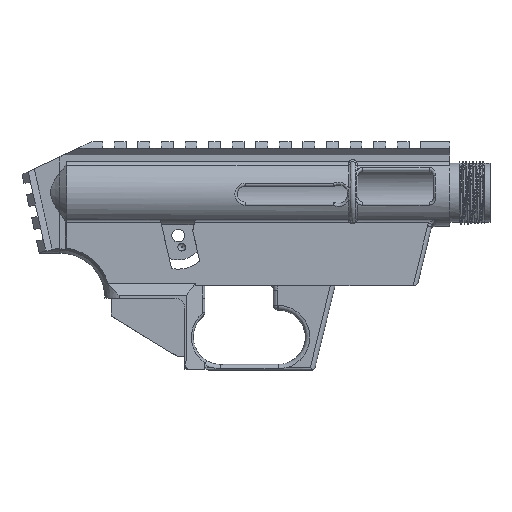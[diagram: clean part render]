
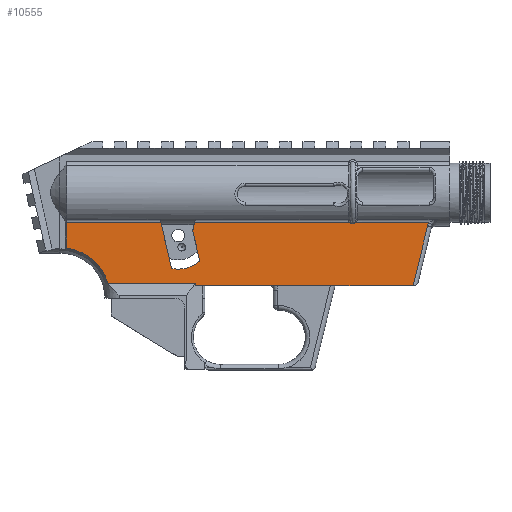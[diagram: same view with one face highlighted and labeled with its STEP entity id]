
A CAD part, left-side view. The second image highlights one B-rep face of the part: STEP entity #10555.
In plain terms, the highlighted planar face has unit normal (-1, 0, 0).
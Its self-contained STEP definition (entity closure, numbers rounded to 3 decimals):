
#199=PLANE('',#11214);
#595=FACE_OUTER_BOUND('',#1184,.T.);
#1184=EDGE_LOOP('',(#7432,#7433,#7434,#7435,#7436,#7437,#7438,#7439,#7440,
#7441,#7442,#7443,#7444,#7445,#7446,#7447));
#1806=CIRCLE('',#11215,14.884);
#1807=CIRCLE('',#11216,22.405);
#2056=B_SPLINE_CURVE_WITH_KNOTS('',3,(#16183,#16184,#16185,#16186,#16187,
#16188,#16189,#16190,#16191,#16192,#16193,#16194),.UNSPECIFIED.,.F.,.F.,
(4,2,2,2,2,4),(0.,0.021,0.047,0.063,
0.077,0.097),.UNSPECIFIED.);
#2060=B_SPLINE_CURVE_WITH_KNOTS('',3,(#16356,#16357,#16358,#16359,#16360,
#16361,#16362,#16363,#16364,#16365,#16366,#16367,#16368),.UNSPECIFIED.,
 .F.,.F.,(4,2,2,3,2,4),(-0.102,-0.09,-0.043,
0.,0.045,0.072),.UNSPECIFIED.);
#2062=B_SPLINE_CURVE_WITH_KNOTS('',3,(#16396,#16397,#16398,#16399,#16400,
#16401),.UNSPECIFIED.,.F.,.F.,(4,2,4),(0.,0.074,0.148),
 .UNSPECIFIED.);
#2259=LINE('',#15268,#3368);
#2299=LINE('',#16375,#3408);
#2300=LINE('',#16377,#3409);
#2301=LINE('',#16379,#3410);
#2302=LINE('',#16383,#3411);
#2303=LINE('',#16385,#3412);
#2304=LINE('',#16387,#3413);
#2305=LINE('',#16391,#3414);
#2306=LINE('',#16392,#3415);
#2307=LINE('',#16394,#3416);
#2308=LINE('',#16402,#3417);
#3368=VECTOR('',#12063,10.);
#3408=VECTOR('',#12255,10.);
#3409=VECTOR('',#12256,10.);
#3410=VECTOR('',#12257,10.);
#3411=VECTOR('',#12260,10.);
#3412=VECTOR('',#12261,10.);
#3413=VECTOR('',#12262,10.);
#3414=VECTOR('',#12265,10.);
#3415=VECTOR('',#12266,10.);
#3416=VECTOR('',#12267,10.);
#3417=VECTOR('',#12268,10.);
#4500=VERTEX_POINT('',#15265);
#4501=VERTEX_POINT('',#15267);
#4616=VERTEX_POINT('',#16181);
#4617=VERTEX_POINT('',#16182);
#4619=VERTEX_POINT('',#16355);
#4620=VERTEX_POINT('',#16374);
#4621=VERTEX_POINT('',#16376);
#4622=VERTEX_POINT('',#16378);
#4623=VERTEX_POINT('',#16380);
#4624=VERTEX_POINT('',#16382);
#4625=VERTEX_POINT('',#16384);
#4626=VERTEX_POINT('',#16386);
#4627=VERTEX_POINT('',#16388);
#4628=VERTEX_POINT('',#16390);
#4629=VERTEX_POINT('',#16393);
#4630=VERTEX_POINT('',#16395);
#5566=EDGE_CURVE('',#4500,#4501,#2259,.T.);
#5710=EDGE_CURVE('',#4616,#4617,#2056,.T.);
#5714=EDGE_CURVE('',#4619,#4616,#2060,.T.);
#5716=EDGE_CURVE('',#4620,#4617,#2299,.T.);
#5717=EDGE_CURVE('',#4621,#4620,#2300,.T.);
#5718=EDGE_CURVE('',#4622,#4621,#2301,.T.);
#5719=EDGE_CURVE('',#4623,#4622,#1806,.T.);
#5720=EDGE_CURVE('',#4624,#4623,#2302,.T.);
#5721=EDGE_CURVE('',#4625,#4624,#2303,.T.);
#5722=EDGE_CURVE('',#4626,#4625,#2304,.T.);
#5723=EDGE_CURVE('',#4627,#4626,#1807,.T.);
#5724=EDGE_CURVE('',#4627,#4628,#2305,.T.);
#5725=EDGE_CURVE('',#4628,#4501,#2306,.T.);
#5726=EDGE_CURVE('',#4629,#4500,#2307,.T.);
#5727=EDGE_CURVE('',#4630,#4629,#2062,.T.);
#5728=EDGE_CURVE('',#4619,#4630,#2308,.T.);
#7432=ORIENTED_EDGE('',*,*,#5710,.T.);
#7433=ORIENTED_EDGE('',*,*,#5716,.F.);
#7434=ORIENTED_EDGE('',*,*,#5717,.F.);
#7435=ORIENTED_EDGE('',*,*,#5718,.F.);
#7436=ORIENTED_EDGE('',*,*,#5719,.F.);
#7437=ORIENTED_EDGE('',*,*,#5720,.F.);
#7438=ORIENTED_EDGE('',*,*,#5721,.F.);
#7439=ORIENTED_EDGE('',*,*,#5722,.F.);
#7440=ORIENTED_EDGE('',*,*,#5723,.F.);
#7441=ORIENTED_EDGE('',*,*,#5724,.T.);
#7442=ORIENTED_EDGE('',*,*,#5725,.T.);
#7443=ORIENTED_EDGE('',*,*,#5566,.F.);
#7444=ORIENTED_EDGE('',*,*,#5726,.F.);
#7445=ORIENTED_EDGE('',*,*,#5727,.F.);
#7446=ORIENTED_EDGE('',*,*,#5728,.F.);
#7447=ORIENTED_EDGE('',*,*,#5714,.T.);
#10555=ADVANCED_FACE('',(#595),#199,.T.);
#11214=AXIS2_PLACEMENT_3D('',#16373,#12253,#12254);
#11215=AXIS2_PLACEMENT_3D('',#16381,#12258,#12259);
#11216=AXIS2_PLACEMENT_3D('',#16389,#12263,#12264);
#12063=DIRECTION('',(0.,1.,0.));
#12253=DIRECTION('center_axis',(-1.,0.,0.));
#12254=DIRECTION('ref_axis',(0.,0.,1.));
#12255=DIRECTION('',(0.,-1.,0.));
#12256=DIRECTION('',(0.,-0.225,0.974));
#12257=DIRECTION('',(0.,0.225,0.974));
#12258=DIRECTION('center_axis',(-1.,0.,0.));
#12259=DIRECTION('ref_axis',(0.,-1.,0.));
#12260=DIRECTION('',(0.,-0.229,-0.973));
#12261=DIRECTION('',(0.,-1.,0.));
#12262=DIRECTION('',(0.,0.,1.));
#12263=DIRECTION('center_axis',(-1.,0.,0.));
#12264=DIRECTION('ref_axis',(0.,0.,1.));
#12265=DIRECTION('',(0.,-1.,0.));
#12266=DIRECTION('',(0.,0.,-1.));
#12267=DIRECTION('',(0.,0.236,-0.972));
#12268=DIRECTION('',(0.,-1.,0.));
#15265=CARTESIAN_POINT('',(-8.42,-61.545,0.));
#15267=CARTESIAN_POINT('',(-8.42,34.978,0.));
#15268=CARTESIAN_POINT('',(-8.42,17.489,0.));
#16181=CARTESIAN_POINT('',(-8.42,-34.046,27.659));
#16182=CARTESIAN_POINT('',(-8.42,-33.329,27.888));
#16183=CARTESIAN_POINT('Ctrl Pts',(-8.42,-34.046,27.659));
#16184=CARTESIAN_POINT('Ctrl Pts',(-8.42,-33.992,27.704));
#16185=CARTESIAN_POINT('Ctrl Pts',(-8.42,-33.933,27.741));
#16186=CARTESIAN_POINT('Ctrl Pts',(-8.42,-33.793,27.81));
#16187=CARTESIAN_POINT('Ctrl Pts',(-8.42,-33.722,27.831));
#16188=CARTESIAN_POINT('Ctrl Pts',(-8.42,-33.629,27.852));
#16189=CARTESIAN_POINT('Ctrl Pts',(-8.42,-33.594,27.859));
#16190=CARTESIAN_POINT('Ctrl Pts',(-8.42,-33.527,27.868));
#16191=CARTESIAN_POINT('Ctrl Pts',(-8.42,-33.495,27.872));
#16192=CARTESIAN_POINT('Ctrl Pts',(-8.42,-33.419,27.88));
#16193=CARTESIAN_POINT('Ctrl Pts',(-8.42,-33.377,27.884));
#16194=CARTESIAN_POINT('Ctrl Pts',(-8.42,-33.329,27.888));
#16355=CARTESIAN_POINT('',(-8.42,-35.664,27.888));
#16356=CARTESIAN_POINT('Ctrl Pts',(-8.42,-35.664,27.888));
#16357=CARTESIAN_POINT('Ctrl Pts',(-8.42,-35.638,27.853));
#16358=CARTESIAN_POINT('Ctrl Pts',(-8.42,-35.61,27.819));
#16359=CARTESIAN_POINT('Ctrl Pts',(-8.42,-35.478,27.674));
#16360=CARTESIAN_POINT('Ctrl Pts',(-8.42,-35.329,27.561));
#16361=CARTESIAN_POINT('Ctrl Pts',(-8.42,-35.057,27.438));
#16362=CARTESIAN_POINT('Ctrl Pts',(-8.42,-34.889,27.401));
#16363=CARTESIAN_POINT('Ctrl Pts',(-8.42,-34.746,27.401));
#16364=CARTESIAN_POINT('Ctrl Pts',(-8.42,-34.597,27.401));
#16365=CARTESIAN_POINT('Ctrl Pts',(-8.42,-34.422,27.442));
#16366=CARTESIAN_POINT('Ctrl Pts',(-8.42,-34.206,27.544));
#16367=CARTESIAN_POINT('Ctrl Pts',(-8.42,-34.122,27.597));
#16368=CARTESIAN_POINT('Ctrl Pts',(-8.42,-34.046,27.659));
#16373=CARTESIAN_POINT('Origin',(-8.42,0.,0.));
#16374=CARTESIAN_POINT('',(-8.42,35.445,27.888));
#16375=CARTESIAN_POINT('',(-8.42,0.,27.888));
#16376=CARTESIAN_POINT('',(-8.42,36.258,24.36));
#16377=CARTESIAN_POINT('',(-8.42,37.307,19.808));
#16378=CARTESIAN_POINT('',(-8.42,33.128,10.797));
#16379=CARTESIAN_POINT('',(-8.42,32.672,8.823));
#16380=CARTESIAN_POINT('',(-8.42,45.62,7.575));
#16381=CARTESIAN_POINT('Origin',(-8.42,42.724,22.175));
#16382=CARTESIAN_POINT('',(-8.42,50.391,27.845));
#16383=CARTESIAN_POINT('',(-8.42,43.577,-1.101));
#16384=CARTESIAN_POINT('',(-8.42,92.25,27.845));
#16385=CARTESIAN_POINT('',(-8.42,0.,27.845));
#16386=CARTESIAN_POINT('',(-8.42,92.25,16.62));
#16387=CARTESIAN_POINT('',(-8.42,92.25,27.235));
#16388=CARTESIAN_POINT('',(-8.42,73.825,0.971));
#16389=CARTESIAN_POINT('Origin',(-8.42,95.25,-5.583));
#16390=CARTESIAN_POINT('',(-8.42,34.978,0.971));
#16391=CARTESIAN_POINT('',(-8.42,29.708,0.971));
#16392=CARTESIAN_POINT('',(-8.42,34.978,0.));
#16393=CARTESIAN_POINT('',(-8.42,-67.981,26.535));
#16394=CARTESIAN_POINT('',(-8.42,-59.885,-6.843));
#16395=CARTESIAN_POINT('',(-8.42,-68.554,27.888));
#16396=CARTESIAN_POINT('Ctrl Pts',(-8.42,-68.554,27.888));
#16397=CARTESIAN_POINT('Ctrl Pts',(-8.42,-68.423,27.68));
#16398=CARTESIAN_POINT('Ctrl Pts',(-8.42,-68.308,27.461));
#16399=CARTESIAN_POINT('Ctrl Pts',(-8.42,-68.116,27.008));
#16400=CARTESIAN_POINT('Ctrl Pts',(-8.42,-68.039,26.774));
#16401=CARTESIAN_POINT('Ctrl Pts',(-8.42,-67.981,26.535));
#16402=CARTESIAN_POINT('',(-8.42,0.,27.888));
